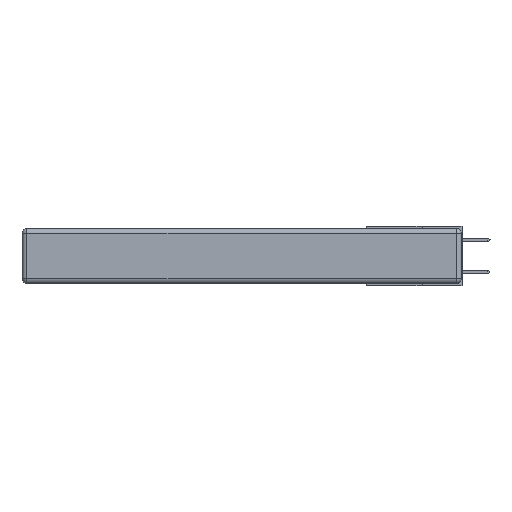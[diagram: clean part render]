
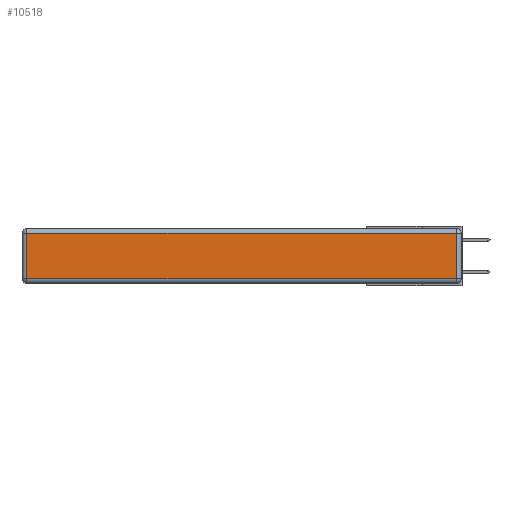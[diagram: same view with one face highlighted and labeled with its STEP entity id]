
A CAD part, left-side view. The second image highlights one B-rep face of the part: STEP entity #10518.
In plain terms, the highlighted planar face has unit normal (-1, 0, 0).
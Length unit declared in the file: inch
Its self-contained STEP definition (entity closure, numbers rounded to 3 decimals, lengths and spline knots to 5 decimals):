
#118 = EDGE_CURVE ( 'NONE', #3480, #4623, #1823, .T. ) ;
#160 = AXIS2_PLACEMENT_3D ( 'NONE', #1292, #10808, #9835 ) ;
#187 = CARTESIAN_POINT ( 'NONE',  ( 0., 0.03, -0.343 ) ) ;
#664 = ORIENTED_EDGE ( 'NONE', *, *, #8180, .T. ) ;
#848 = EDGE_CURVE ( 'NONE', #4103, #3480, #4481, .T. ) ;
#1219 = DIRECTION ( 'NONE',  ( 0., 0., 1. ) ) ;
#1292 = CARTESIAN_POINT ( 'NONE',  ( 0., 0., -0.343 ) ) ;
#1405 = ORIENTED_EDGE ( 'NONE', *, *, #118, .T. ) ;
#1823 = LINE ( 'NONE', #187, #8319 ) ;
#2915 = LINE ( 'NONE', #5518, #6463 ) ;
#3424 = CARTESIAN_POINT ( 'NONE',  ( 0., 2.72, -0.313 ) ) ;
#3480 = VERTEX_POINT ( 'NONE', #10360 ) ;
#3907 = VECTOR ( 'NONE', #11068, 39.37008 ) ;
#4103 = VERTEX_POINT ( 'NONE', #3424 ) ;
#4104 = ORIENTED_EDGE ( 'NONE', *, *, #10838, .T. ) ;
#4481 = LINE ( 'NONE', #6941, #3907 ) ;
#4623 = VERTEX_POINT ( 'NONE', #8711 ) ;
#5307 = ORIENTED_EDGE ( 'NONE', *, *, #848, .T. ) ;
#5518 = CARTESIAN_POINT ( 'NONE',  ( 0., 2.75, -0.03 ) ) ;
#6463 = VECTOR ( 'NONE', #12055, 39.37008 ) ;
#6941 = CARTESIAN_POINT ( 'NONE',  ( 0., 0., -0.313 ) ) ;
#6962 = PLANE ( 'NONE',  #160 ) ;
#7293 = CARTESIAN_POINT ( 'NONE',  ( 0., 2.72, -0.343 ) ) ;
#7538 = LINE ( 'NONE', #7293, #7683 ) ;
#7540 = DIRECTION ( 'NONE',  ( 0., 0., -1. ) ) ;
#7683 = VECTOR ( 'NONE', #7540, 39.37008 ) ;
#8180 = EDGE_CURVE ( 'NONE', #9531, #4103, #7538, .T. ) ;
#8319 = VECTOR ( 'NONE', #1219, 39.37008 ) ;
#8711 = CARTESIAN_POINT ( 'NONE',  ( 0., 0.03, -0.03 ) ) ;
#9124 = FACE_OUTER_BOUND ( 'NONE', #11245, .T. ) ;
#9250 = CARTESIAN_POINT ( 'NONE',  ( 0., 2.72, -0.03 ) ) ;
#9531 = VERTEX_POINT ( 'NONE', #9250 ) ;
#9835 = DIRECTION ( 'NONE',  ( 0., 0., 1. ) ) ;
#10360 = CARTESIAN_POINT ( 'NONE',  ( 0., 0.03, -0.313 ) ) ;
#10518 = ADVANCED_FACE ( 'NONE', ( #9124 ), #6962, .T. ) ;
#10808 = DIRECTION ( 'NONE',  ( -1., 0., 0. ) ) ;
#10838 = EDGE_CURVE ( 'NONE', #4623, #9531, #2915, .T. ) ;
#11068 = DIRECTION ( 'NONE',  ( 0., -1., 0. ) ) ;
#11245 = EDGE_LOOP ( 'NONE', ( #5307, #1405, #4104, #664 ) ) ;
#12055 = DIRECTION ( 'NONE',  ( 0., 1., 0. ) ) ;
